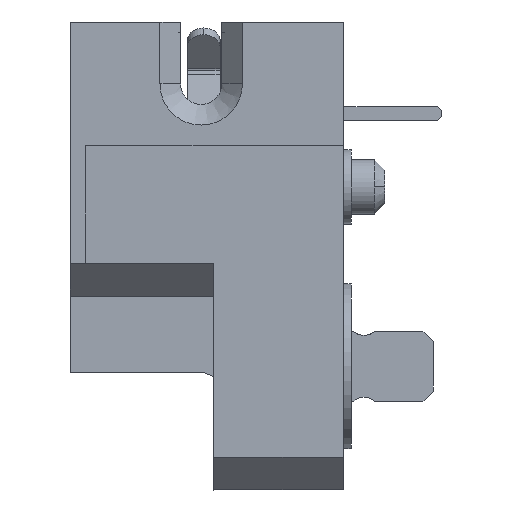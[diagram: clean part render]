
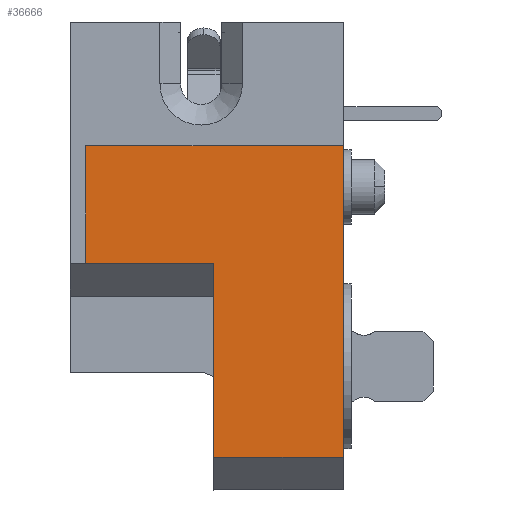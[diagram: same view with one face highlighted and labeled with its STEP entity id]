
A CAD part, left-side view. The second image highlights one B-rep face of the part: STEP entity #36666.
In plain terms, the highlighted planar face has unit normal (-1, 0, 0).
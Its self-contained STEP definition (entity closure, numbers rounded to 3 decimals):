
#2362 = DIRECTION ( 'NONE',  ( 0., -1., 0. ) ) ;
#4424 = VECTOR ( 'NONE', #2362, 1000. ) ;
#9302 = DIRECTION ( 'NONE',  ( 0., 0., 1. ) ) ;
#10034 = LINE ( 'NONE', #40639, #91077 ) ;
#12263 = EDGE_CURVE ( 'NONE', #80290, #69385, #40480, .T. ) ;
#18628 = DIRECTION ( 'NONE',  ( 1., 0., 0. ) ) ;
#18786 = EDGE_CURVE ( 'NONE', #80290, #45992, #44159, .T. ) ;
#18832 = DIRECTION ( 'NONE',  ( 0., -1., 0. ) ) ;
#19281 = CARTESIAN_POINT ( 'NONE',  ( -36.5, 6.25, -2.8 ) ) ;
#19947 = ORIENTED_EDGE ( 'NONE', *, *, #12263, .T. ) ;
#20081 = CARTESIAN_POINT ( 'NONE',  ( -36.5, 0., 0.05 ) ) ;
#21287 = CARTESIAN_POINT ( 'NONE',  ( -36.5, 3.125, -7.5 ) ) ;
#21983 = VECTOR ( 'NONE', #9302, 1000. ) ;
#24665 = CARTESIAN_POINT ( 'NONE',  ( -36.5, 3.125, -3.725 ) ) ;
#25293 = VERTEX_POINT ( 'NONE', #88108 ) ;
#26247 = VERTEX_POINT ( 'NONE', #87577 ) ;
#29568 = DIRECTION ( 'NONE',  ( 0., 0., 1. ) ) ;
#32182 = PLANE ( 'NONE',  #50593 ) ;
#36526 = VECTOR ( 'NONE', #18832, 1000. ) ;
#36666 = ADVANCED_FACE ( 'NONE', ( #49231 ), #32182, .F. ) ;
#37597 = CARTESIAN_POINT ( 'NONE',  ( -36.5, 6.25, -1.375 ) ) ;
#38495 = EDGE_CURVE ( 'NONE', #26247, #69385, #89642, .T. ) ;
#40480 = LINE ( 'NONE', #71078, #4424 ) ;
#40639 = CARTESIAN_POINT ( 'NONE',  ( -36.5, 0., -2.625 ) ) ;
#41091 = EDGE_CURVE ( 'NONE', #45992, #47288, #89061, .T. ) ;
#41633 = EDGE_CURVE ( 'NONE', #25293, #47288, #10034, .T. ) ;
#44159 = LINE ( 'NONE', #37597, #46766 ) ;
#45992 = VERTEX_POINT ( 'NONE', #82281 ) ;
#46766 = VECTOR ( 'NONE', #29568, 1000. ) ;
#47288 = VERTEX_POINT ( 'NONE', #20081 ) ;
#49231 = FACE_OUTER_BOUND ( 'NONE', #68159, .T. ) ;
#50593 = AXIS2_PLACEMENT_3D ( 'NONE', #24665, #18628, #80331 ) ;
#51902 = DIRECTION ( 'NONE',  ( 0., 1., 0. ) ) ;
#55196 = ORIENTED_EDGE ( 'NONE', *, *, #91230, .F. ) ;
#56340 = ORIENTED_EDGE ( 'NONE', *, *, #41091, .F. ) ;
#60447 = ORIENTED_EDGE ( 'NONE', *, *, #41633, .T. ) ;
#63703 = DIRECTION ( 'NONE',  ( 0., 0., 1. ) ) ;
#66428 = VECTOR ( 'NONE', #51902, 1000. ) ;
#67432 = LINE ( 'NONE', #21287, #66428 ) ;
#68159 = EDGE_LOOP ( 'NONE', ( #56340, #73103, #19947, #93304, #55196, #60447 ) ) ;
#68735 = CARTESIAN_POINT ( 'NONE',  ( -36.5, 3.15, -2.8 ) ) ;
#69385 = VERTEX_POINT ( 'NONE', #68735 ) ;
#71078 = CARTESIAN_POINT ( 'NONE',  ( -36.5, 4.89, -2.8 ) ) ;
#73103 = ORIENTED_EDGE ( 'NONE', *, *, #18786, .F. ) ;
#80290 = VERTEX_POINT ( 'NONE', #19281 ) ;
#80331 = DIRECTION ( 'NONE',  ( 0., 0., -1. ) ) ;
#81548 = CARTESIAN_POINT ( 'NONE',  ( -36.5, 3.125, 0.05 ) ) ;
#82124 = CARTESIAN_POINT ( 'NONE',  ( -36.5, 3.15, -3.725 ) ) ;
#82281 = CARTESIAN_POINT ( 'NONE',  ( -36.5, 6.25, 0.05 ) ) ;
#87577 = CARTESIAN_POINT ( 'NONE',  ( -36.5, 3.15, -7.5 ) ) ;
#88108 = CARTESIAN_POINT ( 'NONE',  ( -36.5, 0., -7.5 ) ) ;
#89061 = LINE ( 'NONE', #81548, #36526 ) ;
#89642 = LINE ( 'NONE', #82124, #21983 ) ;
#91077 = VECTOR ( 'NONE', #63703, 1000. ) ;
#91230 = EDGE_CURVE ( 'NONE', #25293, #26247, #67432, .T. ) ;
#93304 = ORIENTED_EDGE ( 'NONE', *, *, #38495, .F. ) ;
